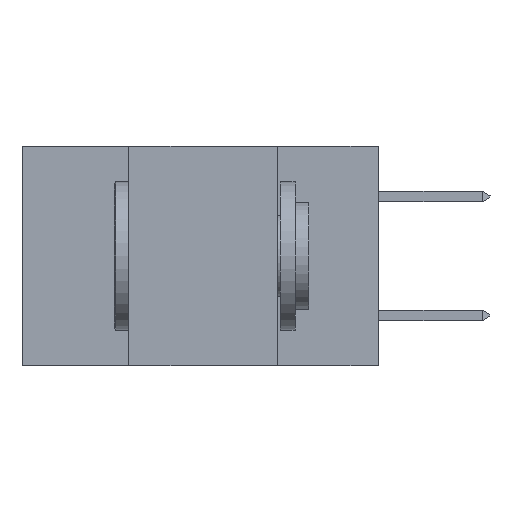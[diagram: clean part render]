
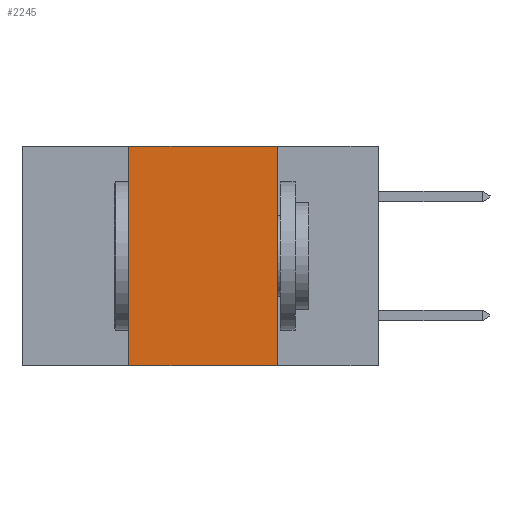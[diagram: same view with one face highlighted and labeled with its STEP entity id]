
A CAD part, left-side view. The second image highlights one B-rep face of the part: STEP entity #2245.
In plain terms, the highlighted planar face has unit normal (-1, 0, 0).
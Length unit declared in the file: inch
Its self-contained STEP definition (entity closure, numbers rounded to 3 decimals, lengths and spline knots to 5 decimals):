
#95 = CARTESIAN_POINT ( 'NONE',  ( 0., 0.42, -0.37 ) ) ;
#107 = FACE_OUTER_BOUND ( 'NONE', #2708, .T. ) ;
#294 = LINE ( 'NONE', #2827, #5254 ) ;
#855 = DIRECTION ( 'NONE',  ( 0., -1., 0. ) ) ;
#1517 = LINE ( 'NONE', #95, #2403 ) ;
#1668 = EDGE_CURVE ( 'NONE', #17322, #5462, #1517, .T. ) ;
#1722 = DIRECTION ( 'NONE',  ( 0., 0., -1. ) ) ;
#1798 = CARTESIAN_POINT ( 'NONE',  ( 0., 0.17, 0. ) ) ;
#2000 = DIRECTION ( 'NONE',  ( 0., -1., 0. ) ) ;
#2245 = ADVANCED_FACE ( 'NONE', ( #107 ), #4224, .F. ) ;
#2403 = VECTOR ( 'NONE', #3053, 39.37008 ) ;
#2708 = EDGE_LOOP ( 'NONE', ( #3965, #7005, #7997, #12353 ) ) ;
#2827 = CARTESIAN_POINT ( 'NONE',  ( 0., 0.17, -0.37 ) ) ;
#3053 = DIRECTION ( 'NONE',  ( 0., 0., 1. ) ) ;
#3066 = DIRECTION ( 'NONE',  ( 0., 0., -1. ) ) ;
#3302 = EDGE_CURVE ( 'NONE', #5462, #8992, #14272, .T. ) ;
#3965 = ORIENTED_EDGE ( 'NONE', *, *, #17050, .F. ) ;
#4224 = PLANE ( 'NONE',  #9317 ) ;
#5254 = VECTOR ( 'NONE', #1722, 39.37008 ) ;
#5462 = VERTEX_POINT ( 'NONE', #15394 ) ;
#6173 = EDGE_CURVE ( 'NONE', #17322, #15352, #17152, .T. ) ;
#7005 = ORIENTED_EDGE ( 'NONE', *, *, #3302, .F. ) ;
#7997 = ORIENTED_EDGE ( 'NONE', *, *, #1668, .F. ) ;
#8266 = VECTOR ( 'NONE', #855, 39.37008 ) ;
#8992 = VERTEX_POINT ( 'NONE', #1798 ) ;
#9317 = AXIS2_PLACEMENT_3D ( 'NONE', #13803, #12551, #3066 ) ;
#10341 = CARTESIAN_POINT ( 'NONE',  ( 0., 0.6, 0. ) ) ;
#11969 = CARTESIAN_POINT ( 'NONE',  ( 0., 0.6, -0.37 ) ) ;
#12353 = ORIENTED_EDGE ( 'NONE', *, *, #6173, .T. ) ;
#12551 = DIRECTION ( 'NONE',  ( 1., 0., 0. ) ) ;
#13630 = CARTESIAN_POINT ( 'NONE',  ( 0., 0.42, -0.37 ) ) ;
#13803 = CARTESIAN_POINT ( 'NONE',  ( 0., 0.6, 0. ) ) ;
#14194 = CARTESIAN_POINT ( 'NONE',  ( 0., 0.17, -0.37 ) ) ;
#14272 = LINE ( 'NONE', #10341, #16726 ) ;
#15352 = VERTEX_POINT ( 'NONE', #14194 ) ;
#15394 = CARTESIAN_POINT ( 'NONE',  ( 0., 0.42, 0. ) ) ;
#16726 = VECTOR ( 'NONE', #2000, 39.37008 ) ;
#17050 = EDGE_CURVE ( 'NONE', #8992, #15352, #294, .T. ) ;
#17152 = LINE ( 'NONE', #11969, #8266 ) ;
#17322 = VERTEX_POINT ( 'NONE', #13630 ) ;
